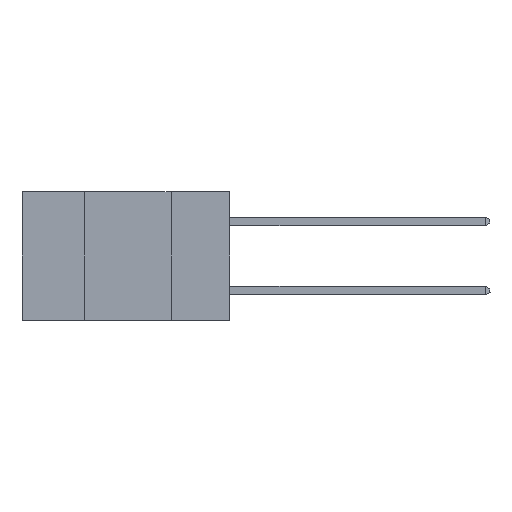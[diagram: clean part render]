
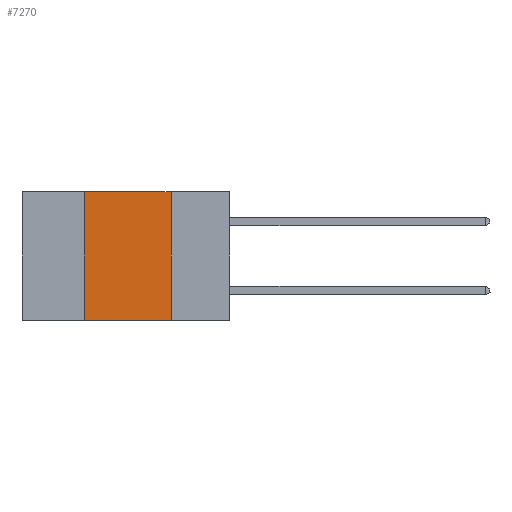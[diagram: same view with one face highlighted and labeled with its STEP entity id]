
A CAD part, left-side view. The second image highlights one B-rep face of the part: STEP entity #7270.
In plain terms, the highlighted planar face has unit normal (-1, 0, 0).
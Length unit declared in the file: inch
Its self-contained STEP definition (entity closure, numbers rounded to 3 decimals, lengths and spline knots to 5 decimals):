
#323 = VERTEX_POINT ( 'NONE', #12147 ) ;
#1715 = CARTESIAN_POINT ( 'NONE',  ( 0., 0.17, 0. ) ) ;
#1784 = CARTESIAN_POINT ( 'NONE',  ( 0., 0.6, 0. ) ) ;
#1865 = ORIENTED_EDGE ( 'NONE', *, *, #8826, .F. ) ;
#1928 = EDGE_LOOP ( 'NONE', ( #4841, #1865, #2343, #4675 ) ) ;
#2104 = VECTOR ( 'NONE', #3079, 39.37008 ) ;
#2343 = ORIENTED_EDGE ( 'NONE', *, *, #11906, .F. ) ;
#2517 = PLANE ( 'NONE',  #9887 ) ;
#2545 = CARTESIAN_POINT ( 'NONE',  ( 0., 0.42, 0. ) ) ;
#2951 = VECTOR ( 'NONE', #11839, 39.37008 ) ;
#3079 = DIRECTION ( 'NONE',  ( 0., 0., 1. ) ) ;
#3131 = LINE ( 'NONE', #5954, #12989 ) ;
#3229 = EDGE_CURVE ( 'NONE', #323, #5926, #3131, .T. ) ;
#4264 = VERTEX_POINT ( 'NONE', #11889 ) ;
#4435 = VECTOR ( 'NONE', #10857, 39.37008 ) ;
#4675 = ORIENTED_EDGE ( 'NONE', *, *, #3229, .T. ) ;
#4841 = ORIENTED_EDGE ( 'NONE', *, *, #11434, .F. ) ;
#5595 = DIRECTION ( 'NONE',  ( 1., 0., 0. ) ) ;
#5926 = VERTEX_POINT ( 'NONE', #10525 ) ;
#5954 = CARTESIAN_POINT ( 'NONE',  ( 0., 0.6, -0.37 ) ) ;
#6355 = CARTESIAN_POINT ( 'NONE',  ( 0., 0.17, 0. ) ) ;
#6540 = FACE_OUTER_BOUND ( 'NONE', #1928, .T. ) ;
#7270 = ADVANCED_FACE ( 'NONE', ( #6540 ), #2517, .F. ) ;
#8826 = EDGE_CURVE ( 'NONE', #4264, #11601, #11053, .T. ) ;
#9576 = CARTESIAN_POINT ( 'NONE',  ( 0., 0.6, 0. ) ) ;
#9887 = AXIS2_PLACEMENT_3D ( 'NONE', #9576, #5595, #10615 ) ;
#10183 = LINE ( 'NONE', #6355, #4435 ) ;
#10525 = CARTESIAN_POINT ( 'NONE',  ( 0., 0.17, -0.37 ) ) ;
#10615 = DIRECTION ( 'NONE',  ( 0., 0., -1. ) ) ;
#10857 = DIRECTION ( 'NONE',  ( 0., 0., -1. ) ) ;
#11053 = LINE ( 'NONE', #1784, #2951 ) ;
#11434 = EDGE_CURVE ( 'NONE', #11601, #5926, #10183, .T. ) ;
#11601 = VERTEX_POINT ( 'NONE', #1715 ) ;
#11839 = DIRECTION ( 'NONE',  ( 0., -1., 0. ) ) ;
#11889 = CARTESIAN_POINT ( 'NONE',  ( 0., 0.42, 0. ) ) ;
#11906 = EDGE_CURVE ( 'NONE', #323, #4264, #12881, .T. ) ;
#12147 = CARTESIAN_POINT ( 'NONE',  ( 0., 0.42, -0.37 ) ) ;
#12881 = LINE ( 'NONE', #2545, #2104 ) ;
#12989 = VECTOR ( 'NONE', #13043, 39.37008 ) ;
#13043 = DIRECTION ( 'NONE',  ( 0., -1., 0. ) ) ;
